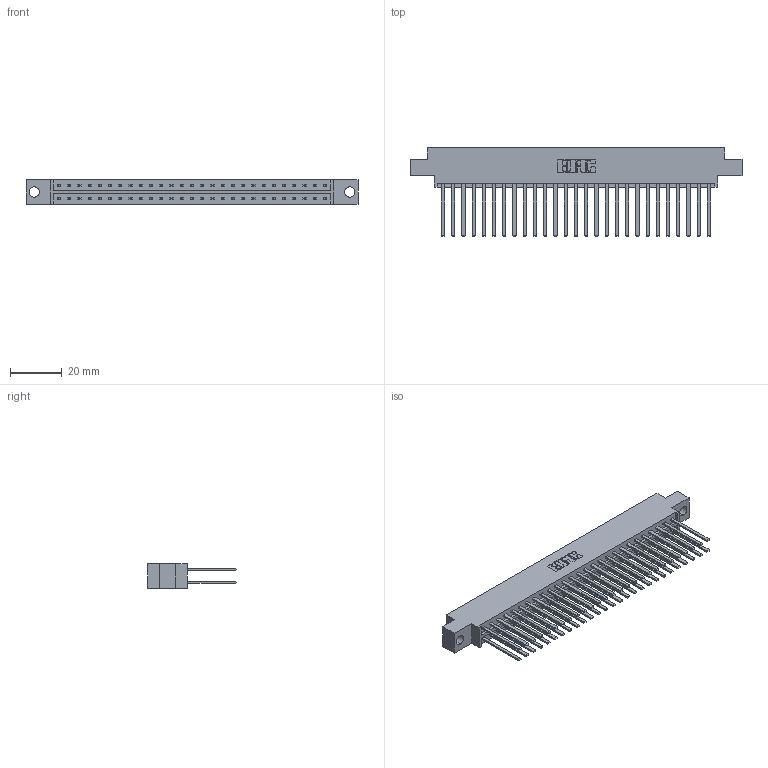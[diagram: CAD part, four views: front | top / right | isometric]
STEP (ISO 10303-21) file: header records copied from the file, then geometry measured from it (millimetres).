
FILE_DESCRIPTION (( 'STEP AP203' ), '1' );
FILE_NAME ('833-054-544-804.STEP', '2020-06-04T21:18:42', ( '' ), ( '' ), 'SwSTEP 2.0', 'SolidWorks 2020', '' );
FILE_SCHEMA (( 'CONFIG_CONTROL_DESIGN' ));
Length unit declared in the file: inch
Products named in the file (3): 833-054-544-804; 345-292-001_345-293-144; 833 Part_Offset - .156 Dia - TH
Assembly tree (55 placements, depth 2):
  833-054-544-804
    833 Part_Offset - .156 Dia - TH
    345-292-001_345-293-144  x54
Bounding box: 128.52 x 34.3 x 9.4 mm (x, y, z)
Volume: 13422.6 mm3; surface area: 18165.2 mm2
Topology: 55 solids, 55 shells, 2602 faces, 7721 edges, 5074 vertices
Faces by surface type: plane 1802, cylinder 800
Entity records: 19261 total; most frequent: CARTESIAN_POINT 3210, ORIENTED_EDGE 3146, DIRECTION 2765, EDGE_CURVE 1573, VECTOR 1449, LINE 1449, VERTEX_POINT 1046, AXIS2_PLACEMENT_3D 658
